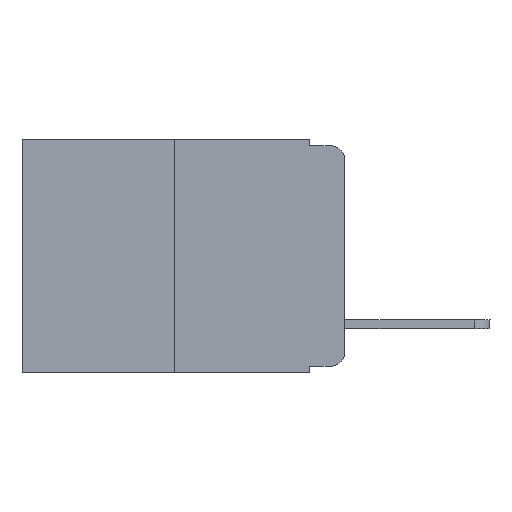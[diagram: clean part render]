
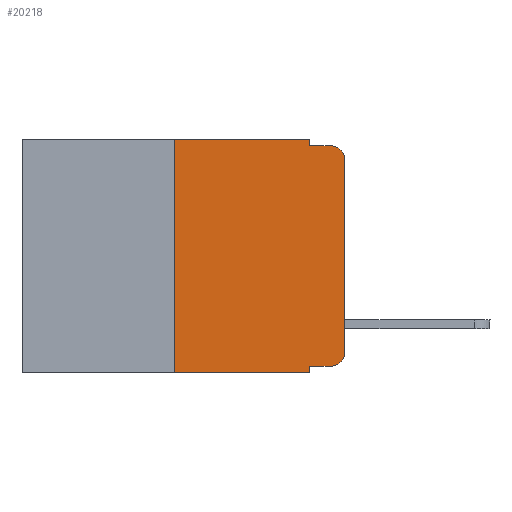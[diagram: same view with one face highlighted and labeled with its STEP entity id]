
A CAD part, left-side view. The second image highlights one B-rep face of the part: STEP entity #20218.
In plain terms, the highlighted planar face has unit normal (-1, 0, 0).
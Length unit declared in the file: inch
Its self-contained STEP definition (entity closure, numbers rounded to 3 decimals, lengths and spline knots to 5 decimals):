
#173 = CARTESIAN_POINT ( 'NONE',  ( 0., 0.473, 0. ) ) ;
#384 = FACE_OUTER_BOUND ( 'NONE', #17396, .T. ) ;
#400 = EDGE_CURVE ( 'NONE', #6808, #5248, #13071, .T. ) ;
#460 = CIRCLE ( 'NONE', #20075, 0.02 ) ;
#580 = CARTESIAN_POINT ( 'NONE',  ( 0., 0.02, -0.333 ) ) ;
#799 = CARTESIAN_POINT ( 'NONE',  ( 0., 0.02, -0.313 ) ) ;
#1666 = VERTEX_POINT ( 'NONE', #15014 ) ;
#1695 = DIRECTION ( 'NONE',  ( 0., -1., 0. ) ) ;
#2003 = DIRECTION ( 'NONE',  ( 0., 0., -1. ) ) ;
#2209 = CARTESIAN_POINT ( 'NONE',  ( 0., 0.051, 0. ) ) ;
#2698 = LINE ( 'NONE', #9277, #10298 ) ;
#3296 = VECTOR ( 'NONE', #8171, 39.37008 ) ;
#3463 = ORIENTED_EDGE ( 'NONE', *, *, #7746, .F. ) ;
#3824 = ORIENTED_EDGE ( 'NONE', *, *, #4727, .T. ) ;
#3846 = CARTESIAN_POINT ( 'NONE',  ( 0., 0.051, 0. ) ) ;
#4029 = CARTESIAN_POINT ( 'NONE',  ( 0., 0.02, -0.03 ) ) ;
#4041 = DIRECTION ( 'NONE',  ( 0., -1., 0. ) ) ;
#4670 = AXIS2_PLACEMENT_3D ( 'NONE', #799, #18474, #20515 ) ;
#4727 = EDGE_CURVE ( 'NONE', #11499, #13587, #5559, .T. ) ;
#4914 = CARTESIAN_POINT ( 'NONE',  ( 0., 0.473, -0.343 ) ) ;
#4979 = CARTESIAN_POINT ( 'NONE',  ( 0., 0.051, -0.333 ) ) ;
#5248 = VERTEX_POINT ( 'NONE', #580 ) ;
#5305 = EDGE_CURVE ( 'NONE', #5248, #11499, #13963, .T. ) ;
#5559 = LINE ( 'NONE', #17197, #8492 ) ;
#5842 = VECTOR ( 'NONE', #4041, 39.37008 ) ;
#6400 = DIRECTION ( 'NONE',  ( 0., -1., 0. ) ) ;
#6808 = VERTEX_POINT ( 'NONE', #9930 ) ;
#6910 = ORIENTED_EDGE ( 'NONE', *, *, #5305, .T. ) ;
#7711 = CARTESIAN_POINT ( 'NONE',  ( 0., 0.051, -0.01 ) ) ;
#7725 = CARTESIAN_POINT ( 'NONE',  ( 0., 0.25, -0.343 ) ) ;
#7746 = EDGE_CURVE ( 'NONE', #6808, #10335, #13652, .T. ) ;
#8171 = DIRECTION ( 'NONE',  ( 0., 0., 1. ) ) ;
#8492 = VECTOR ( 'NONE', #20431, 39.37008 ) ;
#9277 = CARTESIAN_POINT ( 'NONE',  ( 0., 0.051, -0.01 ) ) ;
#9363 = ORIENTED_EDGE ( 'NONE', *, *, #20980, .F. ) ;
#9729 = EDGE_CURVE ( 'NONE', #9975, #10335, #15050, .T. ) ;
#9930 = CARTESIAN_POINT ( 'NONE',  ( 0., 0.051, -0.333 ) ) ;
#9975 = VERTEX_POINT ( 'NONE', #7725 ) ;
#10291 = EDGE_CURVE ( 'NONE', #13587, #20203, #460, .T. ) ;
#10292 = LINE ( 'NONE', #2209, #17055 ) ;
#10298 = VECTOR ( 'NONE', #15840, 39.37008 ) ;
#10335 = VERTEX_POINT ( 'NONE', #20523 ) ;
#10388 = ORIENTED_EDGE ( 'NONE', *, *, #12402, .F. ) ;
#10396 = DIRECTION ( 'NONE',  ( 0., 0., -1. ) ) ;
#10505 = CARTESIAN_POINT ( 'NONE',  ( 0., 0.473, 0. ) ) ;
#10592 = ORIENTED_EDGE ( 'NONE', *, *, #400, .T. ) ;
#10597 = DIRECTION ( 'NONE',  ( 0., 0., -1. ) ) ;
#11499 = VERTEX_POINT ( 'NONE', #18181 ) ;
#11886 = EDGE_CURVE ( 'NONE', #12562, #20203, #2698, .T. ) ;
#12341 = LINE ( 'NONE', #10505, #5842 ) ;
#12402 = EDGE_CURVE ( 'NONE', #1666, #19830, #12341, .T. ) ;
#12520 = ORIENTED_EDGE ( 'NONE', *, *, #10291, .T. ) ;
#12562 = VERTEX_POINT ( 'NONE', #7711 ) ;
#12697 = ORIENTED_EDGE ( 'NONE', *, *, #20470, .F. ) ;
#13017 = LINE ( 'NONE', #14324, #3296 ) ;
#13071 = LINE ( 'NONE', #4979, #18587 ) ;
#13415 = PLANE ( 'NONE',  #18417 ) ;
#13587 = VERTEX_POINT ( 'NONE', #15041 ) ;
#13646 = ORIENTED_EDGE ( 'NONE', *, *, #9729, .T. ) ;
#13652 = LINE ( 'NONE', #3846, #16142 ) ;
#13963 = CIRCLE ( 'NONE', #4670, 0.02 ) ;
#14048 = ORIENTED_EDGE ( 'NONE', *, *, #11886, .F. ) ;
#14324 = CARTESIAN_POINT ( 'NONE',  ( 0., 0.25, 0. ) ) ;
#14924 = DIRECTION ( 'NONE',  ( 1., 0., 0. ) ) ;
#15014 = CARTESIAN_POINT ( 'NONE',  ( 0., 0.25, 0. ) ) ;
#15041 = CARTESIAN_POINT ( 'NONE',  ( 0., 0., -0.03 ) ) ;
#15050 = LINE ( 'NONE', #4914, #16944 ) ;
#15663 = DIRECTION ( 'NONE',  ( 0., 0., -1. ) ) ;
#15840 = DIRECTION ( 'NONE',  ( 0., -1., 0. ) ) ;
#16142 = VECTOR ( 'NONE', #15663, 39.37008 ) ;
#16944 = VECTOR ( 'NONE', #1695, 39.37008 ) ;
#17055 = VECTOR ( 'NONE', #10396, 39.37008 ) ;
#17197 = CARTESIAN_POINT ( 'NONE',  ( 0., 0., 0. ) ) ;
#17396 = EDGE_LOOP ( 'NONE', ( #3824, #12520, #14048, #12697, #10388, #9363, #13646, #3463, #10592, #6910 ) ) ;
#18181 = CARTESIAN_POINT ( 'NONE',  ( 0., 0., -0.313 ) ) ;
#18417 = AXIS2_PLACEMENT_3D ( 'NONE', #173, #14924, #2003 ) ;
#18474 = DIRECTION ( 'NONE',  ( -1., 0., 0. ) ) ;
#18587 = VECTOR ( 'NONE', #6400, 39.37008 ) ;
#18588 = DIRECTION ( 'NONE',  ( -1., 0., 0. ) ) ;
#19669 = CARTESIAN_POINT ( 'NONE',  ( 0., 0.02, -0.01 ) ) ;
#19830 = VERTEX_POINT ( 'NONE', #20583 ) ;
#20075 = AXIS2_PLACEMENT_3D ( 'NONE', #4029, #18588, #10597 ) ;
#20203 = VERTEX_POINT ( 'NONE', #19669 ) ;
#20218 = ADVANCED_FACE ( 'NONE', ( #384 ), #13415, .F. ) ;
#20431 = DIRECTION ( 'NONE',  ( 0., 0., 1. ) ) ;
#20470 = EDGE_CURVE ( 'NONE', #19830, #12562, #10292, .T. ) ;
#20515 = DIRECTION ( 'NONE',  ( 0., 0., -1. ) ) ;
#20523 = CARTESIAN_POINT ( 'NONE',  ( 0., 0.051, -0.343 ) ) ;
#20583 = CARTESIAN_POINT ( 'NONE',  ( 0., 0.051, 0. ) ) ;
#20980 = EDGE_CURVE ( 'NONE', #9975, #1666, #13017, .T. ) ;
